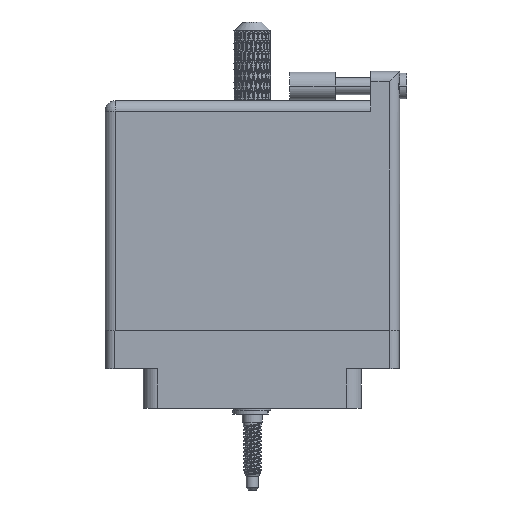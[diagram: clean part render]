
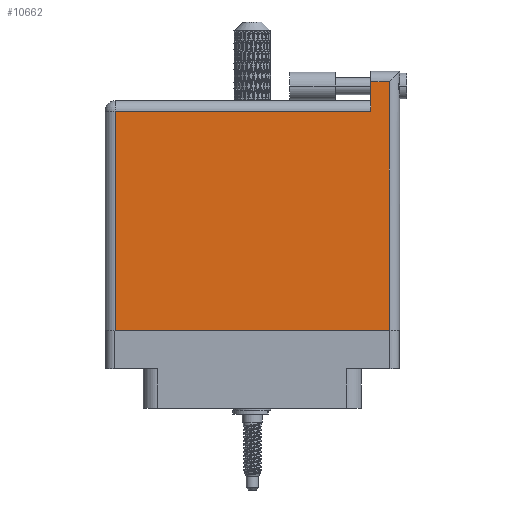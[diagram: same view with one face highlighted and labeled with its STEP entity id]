
A CAD part, front view. The second image highlights one B-rep face of the part: STEP entity #10662.
In plain terms, the highlighted face is planar.
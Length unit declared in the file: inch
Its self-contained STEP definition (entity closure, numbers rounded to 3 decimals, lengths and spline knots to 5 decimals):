
#213 = DIRECTION ( 'NONE',  ( 0., 0., -1. ) ) ;
#3435 = VECTOR ( 'NONE', #99932, 39.37008 ) ;
#3506 = CARTESIAN_POINT ( 'NONE',  ( 1.811, 1.696, 0. ) ) ;
#3584 = EDGE_CURVE ( 'NONE', #42586, #28070, #86787, .T. ) ;
#4487 = FACE_OUTER_BOUND ( 'NONE', #99993, .T. ) ;
#6187 = VERTEX_POINT ( 'NONE', #85931 ) ;
#10485 = ORIENTED_EDGE ( 'NONE', *, *, #3584, .T. ) ;
#10662 = ADVANCED_FACE ( 'NONE', ( #4487 ), #70828, .F. ) ;
#12513 = DIRECTION ( 'NONE',  ( -1., 0., 0. ) ) ;
#14714 = DIRECTION ( 'NONE',  ( 1., 0., 0. ) ) ;
#14925 = CARTESIAN_POINT ( 'NONE',  ( 0.07, 0., 0. ) ) ;
#18227 = EDGE_CURVE ( 'NONE', #21049, #47925, #77154, .T. ) ;
#21049 = VERTEX_POINT ( 'NONE', #3506 ) ;
#24566 = EDGE_CURVE ( 'NONE', #6187, #45652, #48445, .T. ) ;
#24960 = ORIENTED_EDGE ( 'NONE', *, *, #24566, .T. ) ;
#27010 = CARTESIAN_POINT ( 'NONE',  ( 1.811, 1.766, 0. ) ) ;
#28070 = VERTEX_POINT ( 'NONE', #14925 ) ;
#30753 = CARTESIAN_POINT ( 'NONE',  ( 1.938, 1.696, 0. ) ) ;
#33802 = VECTOR ( 'NONE', #12513, 39.37008 ) ;
#37721 = CARTESIAN_POINT ( 'NONE',  ( 1.938, 1.766, 0. ) ) ;
#39458 = CARTESIAN_POINT ( 'NONE',  ( 0., 1.496, 0. ) ) ;
#42586 = VERTEX_POINT ( 'NONE', #100328 ) ;
#42723 = DIRECTION ( 'NONE',  ( 0., -1., 0. ) ) ;
#43877 = AXIS2_PLACEMENT_3D ( 'NONE', #55508, #213, #70183 ) ;
#45652 = VERTEX_POINT ( 'NONE', #30753 ) ;
#46637 = VECTOR ( 'NONE', #92472, 39.37008 ) ;
#47925 = VERTEX_POINT ( 'NONE', #51629 ) ;
#48445 = LINE ( 'NONE', #37721, #3435 ) ;
#51629 = CARTESIAN_POINT ( 'NONE',  ( 1.811, 1.496, 0. ) ) ;
#55508 = CARTESIAN_POINT ( 'NONE',  ( 0., 1.566, 0. ) ) ;
#56800 = EDGE_CURVE ( 'NONE', #28070, #6187, #69573, .T. ) ;
#57456 = DIRECTION ( 'NONE',  ( -1., 0., 0. ) ) ;
#58440 = CARTESIAN_POINT ( 'NONE',  ( 0., 1.696, 0. ) ) ;
#59314 = VECTOR ( 'NONE', #57456, 39.37008 ) ;
#60060 = ORIENTED_EDGE ( 'NONE', *, *, #91743, .T. ) ;
#61968 = CARTESIAN_POINT ( 'NONE',  ( 0., 0., 0. ) ) ;
#69573 = LINE ( 'NONE', #61968, #93912 ) ;
#70183 = DIRECTION ( 'NONE',  ( -1., 0., 0. ) ) ;
#70828 = PLANE ( 'NONE',  #43877 ) ;
#77154 = LINE ( 'NONE', #27010, #78385 ) ;
#78385 = VECTOR ( 'NONE', #42723, 39.37008 ) ;
#79968 = LINE ( 'NONE', #39458, #59314 ) ;
#84978 = CARTESIAN_POINT ( 'NONE',  ( 0.07, 0., 0. ) ) ;
#85931 = CARTESIAN_POINT ( 'NONE',  ( 1.938, 0., 0. ) ) ;
#86787 = LINE ( 'NONE', #84978, #46637 ) ;
#90679 = EDGE_CURVE ( 'NONE', #45652, #21049, #93497, .T. ) ;
#91595 = ORIENTED_EDGE ( 'NONE', *, *, #56800, .T. ) ;
#91743 = EDGE_CURVE ( 'NONE', #47925, #42586, #79968, .T. ) ;
#92472 = DIRECTION ( 'NONE',  ( 0., -1., 0. ) ) ;
#93497 = LINE ( 'NONE', #58440, #33802 ) ;
#93912 = VECTOR ( 'NONE', #14714, 39.37008 ) ;
#97438 = ORIENTED_EDGE ( 'NONE', *, *, #18227, .T. ) ;
#97797 = ORIENTED_EDGE ( 'NONE', *, *, #90679, .T. ) ;
#99932 = DIRECTION ( 'NONE',  ( 0., 1., 0. ) ) ;
#99993 = EDGE_LOOP ( 'NONE', ( #91595, #24960, #97797, #97438, #60060, #10485 ) ) ;
#100328 = CARTESIAN_POINT ( 'NONE',  ( 0.07, 1.496, 0. ) ) ;
